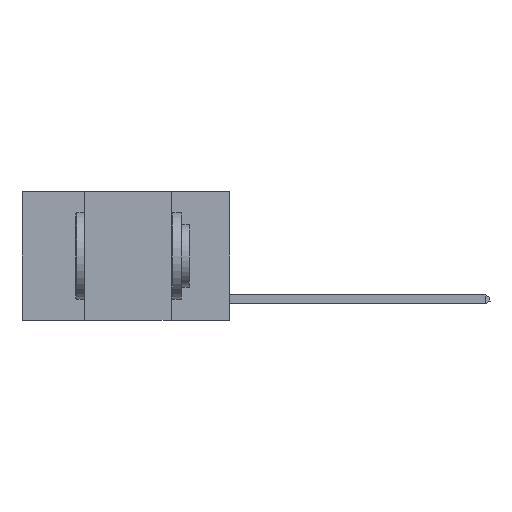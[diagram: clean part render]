
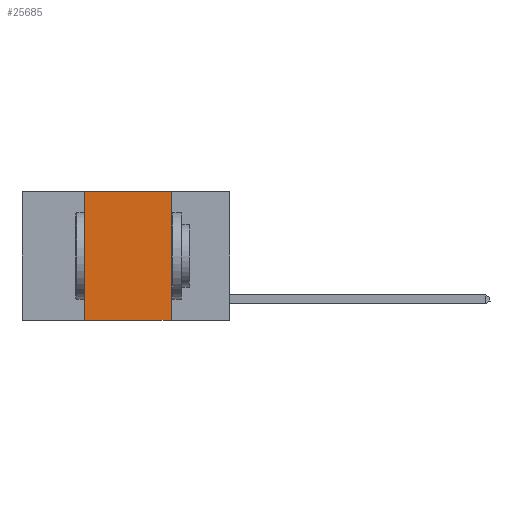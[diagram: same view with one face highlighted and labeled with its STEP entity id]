
A CAD part, left-side view. The second image highlights one B-rep face of the part: STEP entity #25685.
In plain terms, the highlighted planar face has unit normal (-1, 0, 0).
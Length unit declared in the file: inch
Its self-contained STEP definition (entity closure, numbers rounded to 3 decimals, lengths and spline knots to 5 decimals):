
#119 = DIRECTION ( 'NONE',  ( 0., 0., -1. ) ) ;
#275 = ORIENTED_EDGE ( 'NONE', *, *, #6074, .T. ) ;
#885 = CARTESIAN_POINT ( 'NONE',  ( 0., 0.42, 0. ) ) ;
#2587 = DIRECTION ( 'NONE',  ( 0., -1., 0. ) ) ;
#3683 = CARTESIAN_POINT ( 'NONE',  ( 0., 0.17, 0. ) ) ;
#3800 = AXIS2_PLACEMENT_3D ( 'NONE', #17232, #25707, #119 ) ;
#3873 = DIRECTION ( 'NONE',  ( 0., -1., 0. ) ) ;
#4184 = PLANE ( 'NONE',  #3800 ) ;
#6074 = EDGE_CURVE ( 'NONE', #21246, #10209, #25533, .T. ) ;
#7456 = LINE ( 'NONE', #885, #21555 ) ;
#7590 = DIRECTION ( 'NONE',  ( 0., 0., 1. ) ) ;
#8890 = LINE ( 'NONE', #15504, #13854 ) ;
#9274 = ORIENTED_EDGE ( 'NONE', *, *, #16210, .F. ) ;
#10209 = VERTEX_POINT ( 'NONE', #22335 ) ;
#10338 = ORIENTED_EDGE ( 'NONE', *, *, #19178, .F. ) ;
#11437 = VERTEX_POINT ( 'NONE', #26202 ) ;
#12253 = DIRECTION ( 'NONE',  ( 0., 0., -1. ) ) ;
#13854 = VECTOR ( 'NONE', #2587, 39.37008 ) ;
#14397 = CARTESIAN_POINT ( 'NONE',  ( 0., 0.6, -0.37 ) ) ;
#14525 = ORIENTED_EDGE ( 'NONE', *, *, #15879, .F. ) ;
#15504 = CARTESIAN_POINT ( 'NONE',  ( 0., 0.6, 0. ) ) ;
#15879 = EDGE_CURVE ( 'NONE', #23519, #11437, #8890, .T. ) ;
#16210 = EDGE_CURVE ( 'NONE', #11437, #10209, #25065, .T. ) ;
#17232 = CARTESIAN_POINT ( 'NONE',  ( 0., 0.6, 0. ) ) ;
#18519 = VECTOR ( 'NONE', #3873, 39.37008 ) ;
#19178 = EDGE_CURVE ( 'NONE', #21246, #23519, #7456, .T. ) ;
#19200 = FACE_OUTER_BOUND ( 'NONE', #21053, .T. ) ;
#20599 = CARTESIAN_POINT ( 'NONE',  ( 0., 0.42, 0. ) ) ;
#21053 = EDGE_LOOP ( 'NONE', ( #9274, #14525, #10338, #275 ) ) ;
#21246 = VERTEX_POINT ( 'NONE', #24368 ) ;
#21555 = VECTOR ( 'NONE', #7590, 39.37008 ) ;
#22335 = CARTESIAN_POINT ( 'NONE',  ( 0., 0.17, -0.37 ) ) ;
#23519 = VERTEX_POINT ( 'NONE', #20599 ) ;
#24368 = CARTESIAN_POINT ( 'NONE',  ( 0., 0.42, -0.37 ) ) ;
#24959 = VECTOR ( 'NONE', #12253, 39.37008 ) ;
#25065 = LINE ( 'NONE', #3683, #24959 ) ;
#25533 = LINE ( 'NONE', #14397, #18519 ) ;
#25685 = ADVANCED_FACE ( 'NONE', ( #19200 ), #4184, .F. ) ;
#25707 = DIRECTION ( 'NONE',  ( 1., 0., 0. ) ) ;
#26202 = CARTESIAN_POINT ( 'NONE',  ( 0., 0.17, 0. ) ) ;
